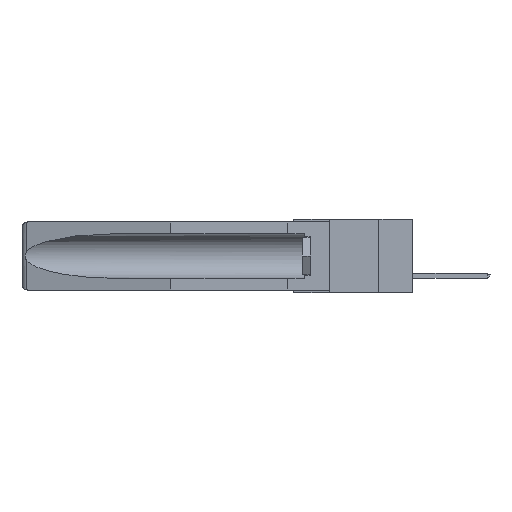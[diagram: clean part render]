
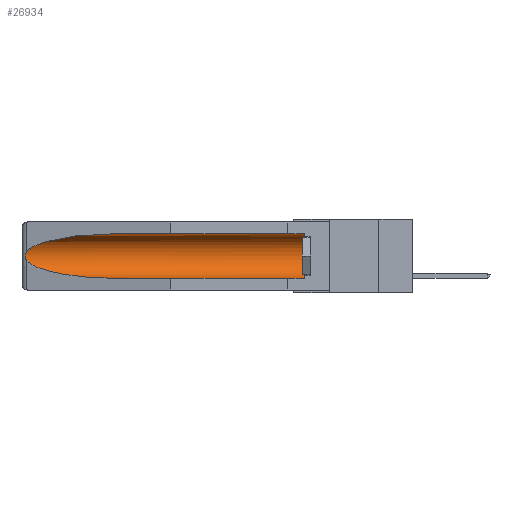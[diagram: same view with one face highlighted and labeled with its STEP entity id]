
A CAD part, left-side view. The second image highlights one B-rep face of the part: STEP entity #26934.
In plain terms, the highlighted cylindrical face has radius 2.857 mm (diameter 5.715 mm), a partial arc.
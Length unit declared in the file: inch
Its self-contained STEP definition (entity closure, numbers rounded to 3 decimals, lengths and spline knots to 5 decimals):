
#1044 = CARTESIAN_POINT ( 'NONE',  ( 0.155, 0.126, -0.059 ) ) ;
#1128 = FACE_OUTER_BOUND ( 'NONE', #4686, .T. ) ;
#1181 = CARTESIAN_POINT ( 'NONE',  ( 0.155, 1.07973, -0.059 ) ) ;
#1575 =( BOUNDED_CURVE ( )  B_SPLINE_CURVE ( 3, ( #1181, #10498, #3620, #20084 ),
 .UNSPECIFIED., .F., .F. ) 
 B_SPLINE_CURVE_WITH_KNOTS ( ( 4, 4 ),
 ( 4.71239, 6.08839 ),
 .UNSPECIFIED. ) 
 CURVE ( )  GEOMETRIC_REPRESENTATION_ITEM ( )  RATIONAL_B_SPLINE_CURVE ( ( 1., 0.848, 0.848, 1. ) ) 
 REPRESENTATION_ITEM ( '' )  );
#1654 = EDGE_CURVE ( 'NONE', #27658, #13142, #5700, .T. ) ;
#2018 = CARTESIAN_POINT ( 'NONE',  ( 0.155, 1.07973, -0.284 ) ) ;
#3458 = VERTEX_POINT ( 'NONE', #20573 ) ;
#3620 = CARTESIAN_POINT ( 'NONE',  ( 0.25451, 1.48313, -0.09465 ) ) ;
#3662 = LINE ( 'NONE', #24176, #8383 ) ;
#4366 = CARTESIAN_POINT ( 'NONE',  ( 0.26537, 1.52718, -0.14972 ) ) ;
#4418 = CARTESIAN_POINT ( 'NONE',  ( 0.155, -0.30754, -0.1715 ) ) ;
#4686 = EDGE_LOOP ( 'NONE', ( #29856, #23561, #5312, #29816, #6397, #7716 ) ) ;
#5085 = CARTESIAN_POINT ( 'NONE',  ( 0.155, 0.126, -0.1715 ) ) ;
#5312 = ORIENTED_EDGE ( 'NONE', *, *, #30045, .T. ) ;
#5700 = CIRCLE ( 'NONE', #17446, 0.1125 ) ;
#5913 = CARTESIAN_POINT ( 'NONE',  ( 0.26537, 1.52718, -0.14972 ) ) ;
#6016 = CARTESIAN_POINT ( 'NONE',  ( 0.26654, 1.53092, -0.15636 ) ) ;
#6121 = CARTESIAN_POINT ( 'NONE',  ( 0.2675, 1.53308, -0.17534 ) ) ;
#6397 = ORIENTED_EDGE ( 'NONE', *, *, #1654, .T. ) ;
#6836 = DIRECTION ( 'NONE',  ( 0., 0., 1. ) ) ;
#7498 = VECTOR ( 'NONE', #27790, 39.37008 ) ;
#7716 = ORIENTED_EDGE ( 'NONE', *, *, #15073, .T. ) ;
#8020 = CYLINDRICAL_SURFACE ( 'NONE', #29531, 0.1125 ) ;
#8373 = CARTESIAN_POINT ( 'NONE',  ( 0.26597, 1.5296, -0.19026 ) ) ;
#8383 = VECTOR ( 'NONE', #19395, 39.37008 ) ;
#8484 = CARTESIAN_POINT ( 'NONE',  ( 0.155, -0.30754, -0.284 ) ) ;
#9497 = EDGE_CURVE ( 'NONE', #29509, #25430, #26727, .T. ) ;
#10498 = CARTESIAN_POINT ( 'NONE',  ( 0.21114, 1.30732, -0.059 ) ) ;
#11771 = CARTESIAN_POINT ( 'NONE',  ( 0.155, 1.07973, -0.059 ) ) ;
#12684 = EDGE_CURVE ( 'NONE', #20987, #29509, #1575, .T. ) ;
#13142 = VERTEX_POINT ( 'NONE', #1044 ) ;
#13774 = CARTESIAN_POINT ( 'NONE',  ( 0.21114, 1.30732, -0.284 ) ) ;
#13855 = DIRECTION ( 'NONE',  ( 0., 1., 0. ) ) ;
#15073 = EDGE_CURVE ( 'NONE', #13142, #20987, #3662, .T. ) ;
#15701 = CARTESIAN_POINT ( 'NONE',  ( 0.155, 0.126, -0.284 ) ) ;
#17446 = AXIS2_PLACEMENT_3D ( 'NONE', #5085, #23695, #28397 ) ;
#17822 = CARTESIAN_POINT ( 'NONE',  ( 0.2673, 1.53269, -0.17917 ) ) ;
#18737 = CARTESIAN_POINT ( 'NONE',  ( 0.26537, 1.52718, -0.19328 ) ) ;
#19395 = DIRECTION ( 'NONE',  ( 0., 1., 0. ) ) ;
#19972 = CARTESIAN_POINT ( 'NONE',  ( 0.26597, 1.52961, -0.15275 ) ) ;
#20084 = CARTESIAN_POINT ( 'NONE',  ( 0.26537, 1.52718, -0.14972 ) ) ;
#20174 = CARTESIAN_POINT ( 'NONE',  ( 0.2673, 1.5327, -0.16383 ) ) ;
#20573 = CARTESIAN_POINT ( 'NONE',  ( 0.155, 1.07973, -0.284 ) ) ;
#20987 = VERTEX_POINT ( 'NONE', #11771 ) ;
#21735 = CARTESIAN_POINT ( 'NONE',  ( 0.26537, 1.52718, -0.19328 ) ) ;
#22090 = CARTESIAN_POINT ( 'NONE',  ( 0.26655, 1.53094, -0.18657 ) ) ;
#22230 =( BOUNDED_CURVE ( )  B_SPLINE_CURVE ( 3, ( #21735, #24094, #13774, #2018 ),
 .UNSPECIFIED., .F., .F. ) 
 B_SPLINE_CURVE_WITH_KNOTS ( ( 4, 4 ),
 ( 0.1948, 1.5708 ),
 .UNSPECIFIED. ) 
 CURVE ( )  GEOMETRIC_REPRESENTATION_ITEM ( )  RATIONAL_B_SPLINE_CURVE ( ( 1., 0.848, 0.848, 1. ) ) 
 REPRESENTATION_ITEM ( '' )  );
#23561 = ORIENTED_EDGE ( 'NONE', *, *, #9497, .T. ) ;
#23598 = EDGE_CURVE ( 'NONE', #27658, #3458, #25371, .T. ) ;
#23695 = DIRECTION ( 'NONE',  ( 0., -1., 0. ) ) ;
#24094 = CARTESIAN_POINT ( 'NONE',  ( 0.25451, 1.48313, -0.24835 ) ) ;
#24176 = CARTESIAN_POINT ( 'NONE',  ( 0.155, -0.30754, -0.059 ) ) ;
#25371 = LINE ( 'NONE', #8484, #7498 ) ;
#25430 = VERTEX_POINT ( 'NONE', #18737 ) ;
#26727 = B_SPLINE_CURVE_WITH_KNOTS ( 'NONE', 3,
 ( #5913, #19972, #6016, #20174, #26982, #6121, #17822, #22090, #8373, #29352 ),
 .UNSPECIFIED., .F., .F.,
 ( 4, 2, 2, 2, 4 ),
 ( 0., 0.00029, 0.00058, 0.00087, 0.00117 ),
 .UNSPECIFIED. ) ;
#26934 = ADVANCED_FACE ( 'NONE', ( #1128 ), #8020, .F. ) ;
#26982 = CARTESIAN_POINT ( 'NONE',  ( 0.2675, 1.53308, -0.16763 ) ) ;
#27658 = VERTEX_POINT ( 'NONE', #15701 ) ;
#27790 = DIRECTION ( 'NONE',  ( 0., 1., 0. ) ) ;
#28397 = DIRECTION ( 'NONE',  ( 0., 0., 1. ) ) ;
#29352 = CARTESIAN_POINT ( 'NONE',  ( 0.26537, 1.52718, -0.19328 ) ) ;
#29509 = VERTEX_POINT ( 'NONE', #4366 ) ;
#29531 = AXIS2_PLACEMENT_3D ( 'NONE', #4418, #13855, #6836 ) ;
#29816 = ORIENTED_EDGE ( 'NONE', *, *, #23598, .F. ) ;
#29856 = ORIENTED_EDGE ( 'NONE', *, *, #12684, .T. ) ;
#30045 = EDGE_CURVE ( 'NONE', #25430, #3458, #22230, .T. ) ;
